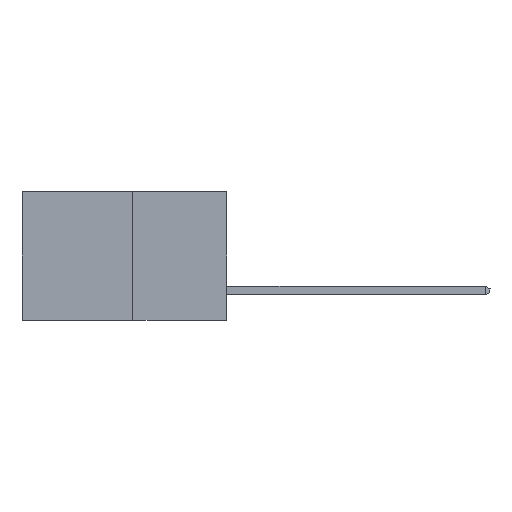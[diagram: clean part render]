
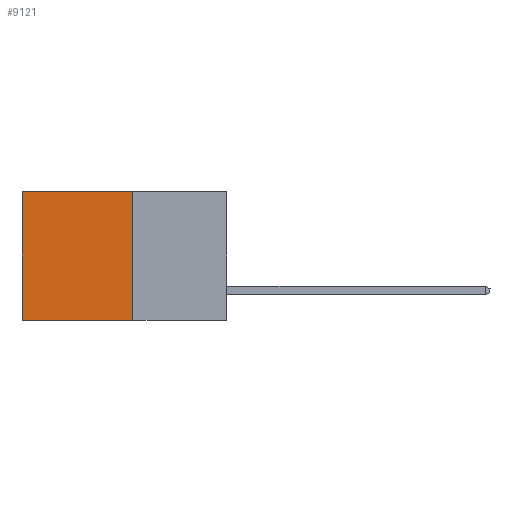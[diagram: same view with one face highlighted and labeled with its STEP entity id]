
A CAD part, left-side view. The second image highlights one B-rep face of the part: STEP entity #9121.
In plain terms, the highlighted planar face has unit normal (-1, 0, 0).
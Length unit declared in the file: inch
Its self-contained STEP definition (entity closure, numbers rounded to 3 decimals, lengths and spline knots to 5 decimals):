
#60 = AXIS2_PLACEMENT_3D ( 'NONE', #1386, #6630, #2227 ) ;
#569 = PLANE ( 'NONE',  #60 ) ;
#905 = ORIENTED_EDGE ( 'NONE', *, *, #1853, .F. ) ;
#1022 = EDGE_CURVE ( 'NONE', #5354, #2928, #1491, .T. ) ;
#1068 = CARTESIAN_POINT ( 'NONE',  ( 0.277, 0.27, -0.37 ) ) ;
#1178 = CARTESIAN_POINT ( 'NONE',  ( 0.277, 0.59, 0. ) ) ;
#1322 = VECTOR ( 'NONE', #5015, 39.37008 ) ;
#1386 = CARTESIAN_POINT ( 'NONE',  ( 0.277, 0.27, -0.37 ) ) ;
#1491 = LINE ( 'NONE', #6722, #7185 ) ;
#1516 = VERTEX_POINT ( 'NONE', #2094 ) ;
#1556 = EDGE_LOOP ( 'NONE', ( #6428, #4224, #905, #4873 ) ) ;
#1853 = EDGE_CURVE ( 'NONE', #1516, #6123, #3502, .T. ) ;
#1935 = DIRECTION ( 'NONE',  ( 0., 1., 0. ) ) ;
#2094 = CARTESIAN_POINT ( 'NONE',  ( 0.277, 0.27, 0. ) ) ;
#2227 = DIRECTION ( 'NONE',  ( 0., 0., -1. ) ) ;
#2928 = VERTEX_POINT ( 'NONE', #8636 ) ;
#3034 = FACE_OUTER_BOUND ( 'NONE', #1556, .T. ) ;
#3502 = LINE ( 'NONE', #5053, #1322 ) ;
#3520 = DIRECTION ( 'NONE',  ( 0., 1., 0. ) ) ;
#3867 = VECTOR ( 'NONE', #1935, 39.37008 ) ;
#4104 = VECTOR ( 'NONE', #3520, 39.37008 ) ;
#4224 = ORIENTED_EDGE ( 'NONE', *, *, #5283, .F. ) ;
#4873 = ORIENTED_EDGE ( 'NONE', *, *, #5291, .T. ) ;
#5015 = DIRECTION ( 'NONE',  ( 0., 0., -1. ) ) ;
#5053 = CARTESIAN_POINT ( 'NONE',  ( 0.277, 0.27, -0.37 ) ) ;
#5283 = EDGE_CURVE ( 'NONE', #6123, #2928, #9075, .T. ) ;
#5291 = EDGE_CURVE ( 'NONE', #1516, #5354, #5803, .T. ) ;
#5354 = VERTEX_POINT ( 'NONE', #1178 ) ;
#5399 = CARTESIAN_POINT ( 'NONE',  ( 0.277, 0.27, -0.37 ) ) ;
#5803 = LINE ( 'NONE', #8306, #4104 ) ;
#6123 = VERTEX_POINT ( 'NONE', #5399 ) ;
#6428 = ORIENTED_EDGE ( 'NONE', *, *, #1022, .T. ) ;
#6630 = DIRECTION ( 'NONE',  ( 1., 0., 0. ) ) ;
#6722 = CARTESIAN_POINT ( 'NONE',  ( 0.277, 0.59, -0.37 ) ) ;
#6764 = DIRECTION ( 'NONE',  ( 0., 0., -1. ) ) ;
#7185 = VECTOR ( 'NONE', #6764, 39.37008 ) ;
#8306 = CARTESIAN_POINT ( 'NONE',  ( 0.277, 0.27, 0. ) ) ;
#8636 = CARTESIAN_POINT ( 'NONE',  ( 0.277, 0.59, -0.37 ) ) ;
#9075 = LINE ( 'NONE', #1068, #3867 ) ;
#9121 = ADVANCED_FACE ( 'NONE', ( #3034 ), #569, .F. ) ;
